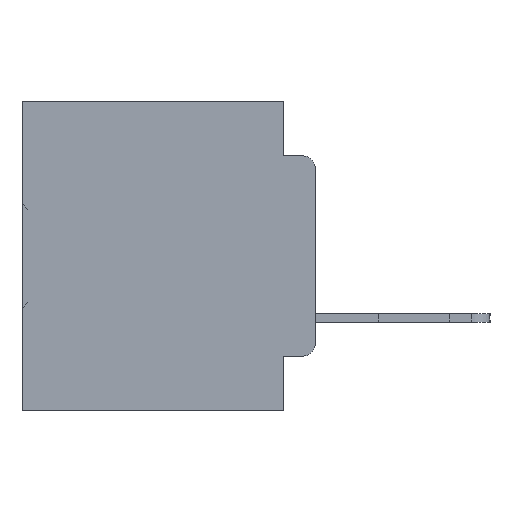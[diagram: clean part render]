
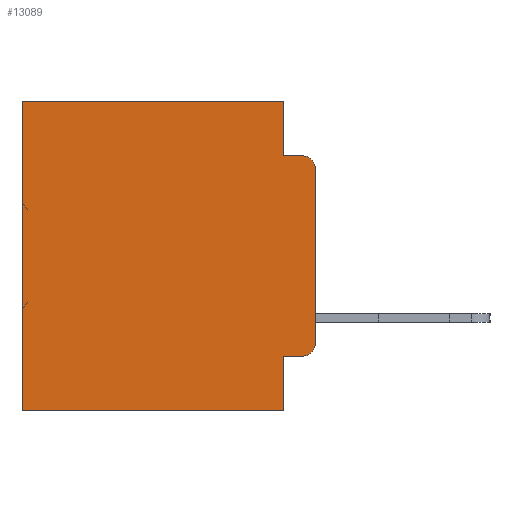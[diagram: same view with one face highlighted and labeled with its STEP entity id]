
A CAD part, left-side view. The second image highlights one B-rep face of the part: STEP entity #13089.
In plain terms, the highlighted planar face has unit normal (-1, 0, 0).
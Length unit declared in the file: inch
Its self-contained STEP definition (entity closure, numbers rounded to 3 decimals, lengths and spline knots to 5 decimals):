
#505 = PLANE ( 'NONE',  #7249 ) ;
#1367 = VECTOR ( 'NONE', #24045, 39.37008 ) ;
#2989 = EDGE_CURVE ( 'NONE', #29172, #32994, #30243, .T. ) ;
#3258 = EDGE_CURVE ( 'NONE', #3384, #15595, #32830, .T. ) ;
#3384 = VERTEX_POINT ( 'NONE', #17845 ) ;
#3517 = DIRECTION ( 'NONE',  ( 0., 0., -1. ) ) ;
#5151 = LINE ( 'NONE', #27971, #27106 ) ;
#5744 = ORIENTED_EDGE ( 'NONE', *, *, #32483, .T. ) ;
#6372 = CARTESIAN_POINT ( 'NONE',  ( 0.298, 0.02, -0.0885 ) ) ;
#6405 = EDGE_CURVE ( 'NONE', #36403, #28079, #36493, .T. ) ;
#6719 = CARTESIAN_POINT ( 'NONE',  ( 0.298, 0.051, -0.4115 ) ) ;
#7080 = ORIENTED_EDGE ( 'NONE', *, *, #33874, .F. ) ;
#7249 = AXIS2_PLACEMENT_3D ( 'NONE', #14882, #20710, #3517 ) ;
#7329 = LINE ( 'NONE', #35203, #13960 ) ;
#7732 = DIRECTION ( 'NONE',  ( 0., 0., -1. ) ) ;
#8932 = CARTESIAN_POINT ( 'NONE',  ( 0.298, 0.02, -0.1085 ) ) ;
#10277 = VECTOR ( 'NONE', #31569, 39.37008 ) ;
#10382 = CARTESIAN_POINT ( 'NONE',  ( 0.298, 0.02, -0.3915 ) ) ;
#10503 = CARTESIAN_POINT ( 'NONE',  ( 0.298, 0.051, -0.4115 ) ) ;
#10575 = ORIENTED_EDGE ( 'NONE', *, *, #2989, .F. ) ;
#11478 = CARTESIAN_POINT ( 'NONE',  ( 0.298, 0.473, 0. ) ) ;
#11715 = CARTESIAN_POINT ( 'NONE',  ( 0.298, 0.02, -0.4115 ) ) ;
#11740 = DIRECTION ( 'NONE',  ( 0., 0., -1. ) ) ;
#11760 = VECTOR ( 'NONE', #12042, 39.37008 ) ;
#12042 = DIRECTION ( 'NONE',  ( 0., -1., 0. ) ) ;
#13089 = ADVANCED_FACE ( 'NONE', ( #26044 ), #505, .F. ) ;
#13245 = DIRECTION ( 'NONE',  ( 0., 0., -1. ) ) ;
#13960 = VECTOR ( 'NONE', #21160, 39.37008 ) ;
#14882 = CARTESIAN_POINT ( 'NONE',  ( 0.298, 0., 0. ) ) ;
#15117 = ORIENTED_EDGE ( 'NONE', *, *, #30634, .T. ) ;
#15125 = DIRECTION ( 'NONE',  ( 0., 1., 0. ) ) ;
#15556 = ORIENTED_EDGE ( 'NONE', *, *, #24925, .F. ) ;
#15595 = VERTEX_POINT ( 'NONE', #24202 ) ;
#15700 = AXIS2_PLACEMENT_3D ( 'NONE', #8932, #29004, #11740 ) ;
#15742 = CIRCLE ( 'NONE', #15700, 0.02 ) ;
#15948 = EDGE_CURVE ( 'NONE', #19635, #32994, #17974, .T. ) ;
#15949 = CARTESIAN_POINT ( 'NONE',  ( 0.298, 0.051, 0. ) ) ;
#16436 = ORIENTED_EDGE ( 'NONE', *, *, #15948, .T. ) ;
#16619 = LINE ( 'NONE', #6719, #1367 ) ;
#17368 = ORIENTED_EDGE ( 'NONE', *, *, #29798, .T. ) ;
#17845 = CARTESIAN_POINT ( 'NONE',  ( 0.298, 0., -0.1085 ) ) ;
#17852 = DIRECTION ( 'NONE',  ( 0., 0., -1. ) ) ;
#17974 = LINE ( 'NONE', #11478, #10277 ) ;
#18325 = CARTESIAN_POINT ( 'NONE',  ( 0.298, 0.051, -0.5 ) ) ;
#19521 = LINE ( 'NONE', #26436, #11760 ) ;
#19635 = VERTEX_POINT ( 'NONE', #24286 ) ;
#20520 = ORIENTED_EDGE ( 'NONE', *, *, #6405, .F. ) ;
#20710 = DIRECTION ( 'NONE',  ( 1., 0., 0. ) ) ;
#21160 = DIRECTION ( 'NONE',  ( 0., 1., 0. ) ) ;
#22706 = VECTOR ( 'NONE', #15125, 39.37008 ) ;
#23176 = AXIS2_PLACEMENT_3D ( 'NONE', #10382, #30475, #13245 ) ;
#23909 = EDGE_LOOP ( 'NONE', ( #27639, #32074, #7080, #20520, #17368, #16436, #10575, #15556, #15117, #5744 ) ) ;
#23939 = CARTESIAN_POINT ( 'NONE',  ( 0.298, 0.051, 0. ) ) ;
#24045 = DIRECTION ( 'NONE',  ( 0., -1., 0. ) ) ;
#24202 = CARTESIAN_POINT ( 'NONE',  ( 0.298, 0., -0.3915 ) ) ;
#24286 = CARTESIAN_POINT ( 'NONE',  ( 0.298, 0.473, 0. ) ) ;
#24871 = VERTEX_POINT ( 'NONE', #10503 ) ;
#24925 = EDGE_CURVE ( 'NONE', #24871, #29172, #5151, .T. ) ;
#25342 = VECTOR ( 'NONE', #17852, 39.37008 ) ;
#26044 = FACE_OUTER_BOUND ( 'NONE', #23909, .T. ) ;
#26336 = EDGE_CURVE ( 'NONE', #3384, #31735, #15742, .T. ) ;
#26436 = CARTESIAN_POINT ( 'NONE',  ( 0.298, 0.051, -0.0885 ) ) ;
#27106 = VECTOR ( 'NONE', #30731, 39.37008 ) ;
#27244 = CARTESIAN_POINT ( 'NONE',  ( 0.298, 0.051, -0.0885 ) ) ;
#27639 = ORIENTED_EDGE ( 'NONE', *, *, #3258, .F. ) ;
#27743 = CIRCLE ( 'NONE', #23176, 0.02 ) ;
#27971 = CARTESIAN_POINT ( 'NONE',  ( 0.298, 0.051, 0. ) ) ;
#28079 = VERTEX_POINT ( 'NONE', #27244 ) ;
#29004 = DIRECTION ( 'NONE',  ( -1., 0., 0. ) ) ;
#29068 = VECTOR ( 'NONE', #7732, 39.37008 ) ;
#29172 = VERTEX_POINT ( 'NONE', #18325 ) ;
#29798 = EDGE_CURVE ( 'NONE', #36403, #19635, #7329, .T. ) ;
#30243 = LINE ( 'NONE', #33316, #22706 ) ;
#30475 = DIRECTION ( 'NONE',  ( -1., 0., 0. ) ) ;
#30634 = EDGE_CURVE ( 'NONE', #24871, #36767, #16619, .T. ) ;
#30731 = DIRECTION ( 'NONE',  ( 0., 0., -1. ) ) ;
#31569 = DIRECTION ( 'NONE',  ( 0., 0., -1. ) ) ;
#31735 = VERTEX_POINT ( 'NONE', #6372 ) ;
#32074 = ORIENTED_EDGE ( 'NONE', *, *, #26336, .T. ) ;
#32483 = EDGE_CURVE ( 'NONE', #36767, #15595, #27743, .T. ) ;
#32830 = LINE ( 'NONE', #33268, #25342 ) ;
#32994 = VERTEX_POINT ( 'NONE', #33370 ) ;
#33268 = CARTESIAN_POINT ( 'NONE',  ( 0.298, 0., 0. ) ) ;
#33316 = CARTESIAN_POINT ( 'NONE',  ( 0.298, 0., -0.5 ) ) ;
#33370 = CARTESIAN_POINT ( 'NONE',  ( 0.298, 0.473, -0.5 ) ) ;
#33874 = EDGE_CURVE ( 'NONE', #28079, #31735, #19521, .T. ) ;
#35203 = CARTESIAN_POINT ( 'NONE',  ( 0.298, 0., 0. ) ) ;
#36403 = VERTEX_POINT ( 'NONE', #23939 ) ;
#36493 = LINE ( 'NONE', #15949, #29068 ) ;
#36767 = VERTEX_POINT ( 'NONE', #11715 ) ;
